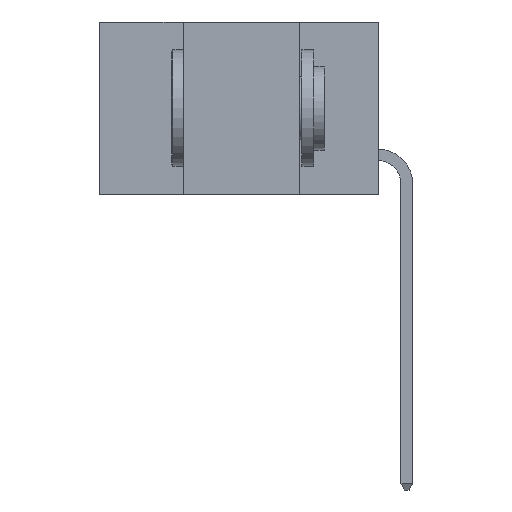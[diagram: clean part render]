
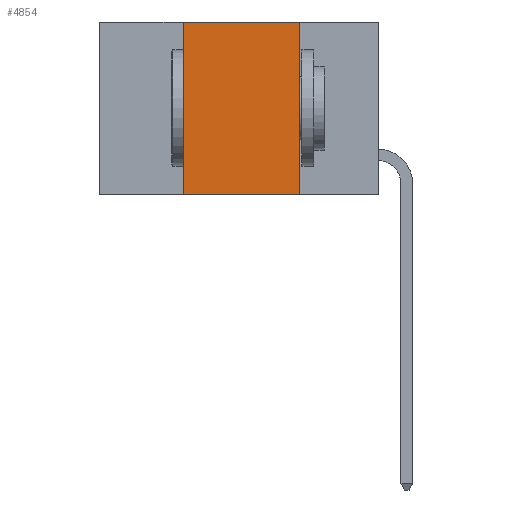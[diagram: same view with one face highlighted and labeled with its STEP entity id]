
A CAD part, left-side view. The second image highlights one B-rep face of the part: STEP entity #4854.
In plain terms, the highlighted planar face has unit normal (-1, 0, 0).
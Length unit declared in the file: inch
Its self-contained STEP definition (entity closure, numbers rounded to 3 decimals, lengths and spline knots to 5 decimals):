
#1001 = AXIS2_PLACEMENT_3D ( 'NONE', #9594, #11867, #6190 ) ;
#1524 = EDGE_CURVE ( 'NONE', #8938, #12982, #7499, .T. ) ;
#1834 = CARTESIAN_POINT ( 'NONE',  ( 0., 0.17, -0.37 ) ) ;
#2419 = VERTEX_POINT ( 'NONE', #6493 ) ;
#2582 = DIRECTION ( 'NONE',  ( 0., 0., 1. ) ) ;
#2707 = ORIENTED_EDGE ( 'NONE', *, *, #8411, .T. ) ;
#3131 = LINE ( 'NONE', #4965, #8728 ) ;
#3592 = EDGE_CURVE ( 'NONE', #2419, #8938, #13828, .T. ) ;
#3805 = PLANE ( 'NONE',  #1001 ) ;
#4092 = DIRECTION ( 'NONE',  ( 0., -1., 0. ) ) ;
#4369 = CARTESIAN_POINT ( 'NONE',  ( 0., 0.17, 0. ) ) ;
#4584 = ORIENTED_EDGE ( 'NONE', *, *, #3592, .F. ) ;
#4681 = CARTESIAN_POINT ( 'NONE',  ( 0., 0.17, -0.37 ) ) ;
#4854 = ADVANCED_FACE ( 'NONE', ( #12339 ), #3805, .F. ) ;
#4965 = CARTESIAN_POINT ( 'NONE',  ( 0., 0.42, -0.37 ) ) ;
#6190 = DIRECTION ( 'NONE',  ( 0., 0., -1. ) ) ;
#6493 = CARTESIAN_POINT ( 'NONE',  ( 0., 0.42, 0. ) ) ;
#7240 = ORIENTED_EDGE ( 'NONE', *, *, #12048, .F. ) ;
#7271 = CARTESIAN_POINT ( 'NONE',  ( 0., 0.6, 0. ) ) ;
#7499 = LINE ( 'NONE', #1834, #7843 ) ;
#7843 = VECTOR ( 'NONE', #11391, 39.37008 ) ;
#7872 = EDGE_LOOP ( 'NONE', ( #10901, #4584, #7240, #2707 ) ) ;
#7987 = VERTEX_POINT ( 'NONE', #11927 ) ;
#8411 = EDGE_CURVE ( 'NONE', #7987, #12982, #14017, .T. ) ;
#8442 = VECTOR ( 'NONE', #4092, 39.37008 ) ;
#8728 = VECTOR ( 'NONE', #2582, 39.37008 ) ;
#8934 = VECTOR ( 'NONE', #9611, 39.37008 ) ;
#8938 = VERTEX_POINT ( 'NONE', #4369 ) ;
#9594 = CARTESIAN_POINT ( 'NONE',  ( 0., 0.6, 0. ) ) ;
#9611 = DIRECTION ( 'NONE',  ( 0., -1., 0. ) ) ;
#9781 = CARTESIAN_POINT ( 'NONE',  ( 0., 0.6, -0.37 ) ) ;
#10901 = ORIENTED_EDGE ( 'NONE', *, *, #1524, .F. ) ;
#11391 = DIRECTION ( 'NONE',  ( 0., 0., -1. ) ) ;
#11867 = DIRECTION ( 'NONE',  ( 1., 0., 0. ) ) ;
#11927 = CARTESIAN_POINT ( 'NONE',  ( 0., 0.42, -0.37 ) ) ;
#12048 = EDGE_CURVE ( 'NONE', #7987, #2419, #3131, .T. ) ;
#12339 = FACE_OUTER_BOUND ( 'NONE', #7872, .T. ) ;
#12982 = VERTEX_POINT ( 'NONE', #4681 ) ;
#13828 = LINE ( 'NONE', #7271, #8934 ) ;
#14017 = LINE ( 'NONE', #9781, #8442 ) ;
